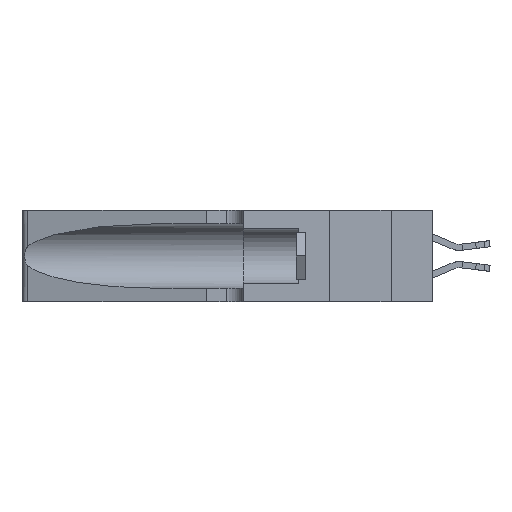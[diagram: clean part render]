
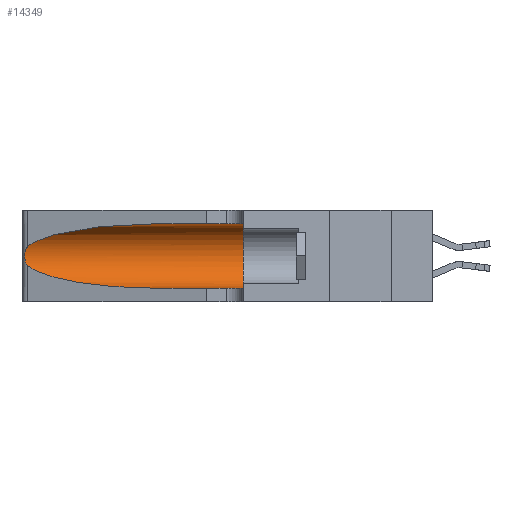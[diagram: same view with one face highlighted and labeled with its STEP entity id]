
A CAD part, left-side view. The second image highlights one B-rep face of the part: STEP entity #14349.
In plain terms, the highlighted cylindrical face has radius 3.308 mm (diameter 6.617 mm), a partial arc.
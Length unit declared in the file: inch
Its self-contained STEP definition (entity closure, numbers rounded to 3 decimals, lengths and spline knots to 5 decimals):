
#386 = VERTEX_POINT ( 'NONE', #7876 ) ;
#1001 = CARTESIAN_POINT ( 'NONE',  ( 0.26075, 1.23896, 0.19203 ) ) ;
#1345 = CARTESIAN_POINT ( 'NONE',  ( 0.2373, 1.15595, 0.08982 ) ) ;
#1375 = EDGE_CURVE ( 'NONE', #13954, #3746, #3346, .T. ) ;
#1406 = CARTESIAN_POINT ( 'NONE',  ( 0.1305, 1.61858, 0.185 ) ) ;
#2183 = EDGE_CURVE ( 'NONE', #386, #3746, #3056, .T. ) ;
#2184 = AXIS2_PLACEMENT_3D ( 'NONE', #1406, #7901, #6325 ) ;
#2656 = CARTESIAN_POINT ( 'NONE',  ( 0.1305, 1.61858, 0.31525 ) ) ;
#2664 = CARTESIAN_POINT ( 'NONE',  ( 0.25555, 1.22994, 0.2215 ) ) ;
#2706 = ORIENTED_EDGE ( 'NONE', *, *, #8214, .T. ) ;
#2742 = CARTESIAN_POINT ( 'NONE',  ( 0.26017, 1.23833, 0.17102 ) ) ;
#2762 =( BOUNDED_CURVE ( )  B_SPLINE_CURVE ( 3, ( #12092, #13669, #4170, #15262 ),
 .UNSPECIFIED., .F., .F. ) 
 B_SPLINE_CURVE_WITH_KNOTS ( ( 4, 4 ),
 ( 1.5708, 2.84003 ),
 .UNSPECIFIED. ) 
 CURVE ( )  GEOMETRIC_REPRESENTATION_ITEM ( )  RATIONAL_B_SPLINE_CURVE ( ( 1., 0.87, 0.87, 1. ) ) 
 REPRESENTATION_ITEM ( '' )  );
#3037 =( BOUNDED_CURVE ( )  B_SPLINE_CURVE ( 3, ( #20384, #1345, #3087, #14184 ),
 .UNSPECIFIED., .F., .F. ) 
 B_SPLINE_CURVE_WITH_KNOTS ( ( 4, 4 ),
 ( 3.44316, 4.71239 ),
 .UNSPECIFIED. ) 
 CURVE ( )  GEOMETRIC_REPRESENTATION_ITEM ( )  RATIONAL_B_SPLINE_CURVE ( ( 1., 0.87, 0.87, 1. ) ) 
 REPRESENTATION_ITEM ( '' )  );
#3056 = LINE ( 'NONE', #16006, #14725 ) ;
#3087 = CARTESIAN_POINT ( 'NONE',  ( 0.18966, 0.96281, 0.05475 ) ) ;
#3123 = CYLINDRICAL_SURFACE ( 'NONE', #2184, 0.13025 ) ;
#3237 = ORIENTED_EDGE ( 'NONE', *, *, #1375, .F. ) ;
#3346 = CIRCLE ( 'NONE', #11864, 0.13025 ) ;
#3421 = B_SPLINE_CURVE_WITH_KNOTS ( 'NONE', 3,
 ( #13776, #2664, #18500, #9061, #20064, #10662, #1001, #12262, #2742, #13842, #4343, #15426, #5933, #16998 ),
 .UNSPECIFIED., .F., .F.,
 ( 4, 2, 2, 2, 2, 2, 4 ),
 ( 0., 0.00027, 0.00053, 0.00107, 0.0016, 0.00187, 0.00214 ),
 .UNSPECIFIED. ) ;
#3430 = CARTESIAN_POINT ( 'NONE',  ( 0.1305, 0.35, 0.05475 ) ) ;
#3746 = VERTEX_POINT ( 'NONE', #3430 ) ;
#4141 = VERTEX_POINT ( 'NONE', #5891 ) ;
#4170 = CARTESIAN_POINT ( 'NONE',  ( 0.2373, 1.15595, 0.28018 ) ) ;
#4343 = CARTESIAN_POINT ( 'NONE',  ( 0.25789, 1.23486, 0.15765 ) ) ;
#5891 = CARTESIAN_POINT ( 'NONE',  ( 0.25487, 1.22718, 0.22369 ) ) ;
#5933 = CARTESIAN_POINT ( 'NONE',  ( 0.25555, 1.22993, 0.14849 ) ) ;
#5937 = ORIENTED_EDGE ( 'NONE', *, *, #7543, .T. ) ;
#6258 = VECTOR ( 'NONE', #7444, 39.37008 ) ;
#6325 = DIRECTION ( 'NONE',  ( 0., 0., -1. ) ) ;
#6893 = CARTESIAN_POINT ( 'NONE',  ( 0.1305, 0.72297, 0.31525 ) ) ;
#6947 = ORIENTED_EDGE ( 'NONE', *, *, #2183, .T. ) ;
#7444 = DIRECTION ( 'NONE',  ( 0., -1., 0. ) ) ;
#7543 = EDGE_CURVE ( 'NONE', #4141, #9060, #3421, .T. ) ;
#7876 = CARTESIAN_POINT ( 'NONE',  ( 0.1305, 0.72297, 0.05475 ) ) ;
#7901 = DIRECTION ( 'NONE',  ( 0., -1., 0. ) ) ;
#8214 = EDGE_CURVE ( 'NONE', #9060, #386, #3037, .T. ) ;
#8279 = EDGE_LOOP ( 'NONE', ( #8654, #5937, #2706, #6947, #3237, #17321 ) ) ;
#8609 = EDGE_CURVE ( 'NONE', #16352, #4141, #2762, .T. ) ;
#8654 = ORIENTED_EDGE ( 'NONE', *, *, #8609, .T. ) ;
#8834 = DIRECTION ( 'NONE',  ( 0., 0., 1. ) ) ;
#8874 = DIRECTION ( 'NONE',  ( 0., 1., 0. ) ) ;
#8883 = CARTESIAN_POINT ( 'NONE',  ( 0.1305, 0.35, 0.185 ) ) ;
#9018 = EDGE_CURVE ( 'NONE', #16352, #13954, #17873, .T. ) ;
#9060 = VERTEX_POINT ( 'NONE', #20116 ) ;
#9061 = CARTESIAN_POINT ( 'NONE',  ( 0.25787, 1.23484, 0.2124 ) ) ;
#10662 = CARTESIAN_POINT ( 'NONE',  ( 0.26018, 1.23835, 0.19895 ) ) ;
#11830 = CARTESIAN_POINT ( 'NONE',  ( 0.1305, 0.35, 0.31525 ) ) ;
#11864 = AXIS2_PLACEMENT_3D ( 'NONE', #8883, #8874, #8834 ) ;
#12092 = CARTESIAN_POINT ( 'NONE',  ( 0.1305, 0.72297, 0.31525 ) ) ;
#12262 = CARTESIAN_POINT ( 'NONE',  ( 0.26075, 1.23896, 0.178 ) ) ;
#13669 = CARTESIAN_POINT ( 'NONE',  ( 0.18966, 0.96281, 0.31525 ) ) ;
#13776 = CARTESIAN_POINT ( 'NONE',  ( 0.25487, 1.22718, 0.22369 ) ) ;
#13842 = CARTESIAN_POINT ( 'NONE',  ( 0.25856, 1.23593, 0.16098 ) ) ;
#13954 = VERTEX_POINT ( 'NONE', #11830 ) ;
#14184 = CARTESIAN_POINT ( 'NONE',  ( 0.1305, 0.72297, 0.05475 ) ) ;
#14349 = ADVANCED_FACE ( 'NONE', ( #19897 ), #3123, .F. ) ;
#14725 = VECTOR ( 'NONE', #16321, 39.37008 ) ;
#15262 = CARTESIAN_POINT ( 'NONE',  ( 0.25487, 1.22718, 0.22369 ) ) ;
#15426 = CARTESIAN_POINT ( 'NONE',  ( 0.25639, 1.23186, 0.15144 ) ) ;
#16006 = CARTESIAN_POINT ( 'NONE',  ( 0.1305, 1.61858, 0.05475 ) ) ;
#16321 = DIRECTION ( 'NONE',  ( 0., -1., 0. ) ) ;
#16352 = VERTEX_POINT ( 'NONE', #6893 ) ;
#16998 = CARTESIAN_POINT ( 'NONE',  ( 0.25487, 1.22718, 0.14631 ) ) ;
#17321 = ORIENTED_EDGE ( 'NONE', *, *, #9018, .F. ) ;
#17873 = LINE ( 'NONE', #2656, #6258 ) ;
#18500 = CARTESIAN_POINT ( 'NONE',  ( 0.25639, 1.23184, 0.21858 ) ) ;
#19897 = FACE_OUTER_BOUND ( 'NONE', #8279, .T. ) ;
#20064 = CARTESIAN_POINT ( 'NONE',  ( 0.25854, 1.2359, 0.20912 ) ) ;
#20116 = CARTESIAN_POINT ( 'NONE',  ( 0.25487, 1.22718, 0.14631 ) ) ;
#20384 = CARTESIAN_POINT ( 'NONE',  ( 0.25487, 1.22718, 0.14631 ) ) ;
